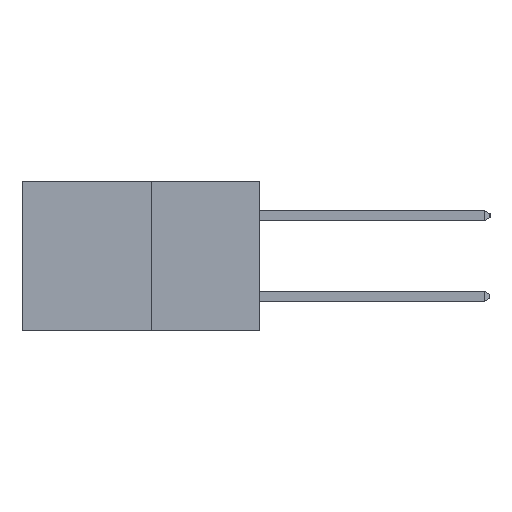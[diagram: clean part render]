
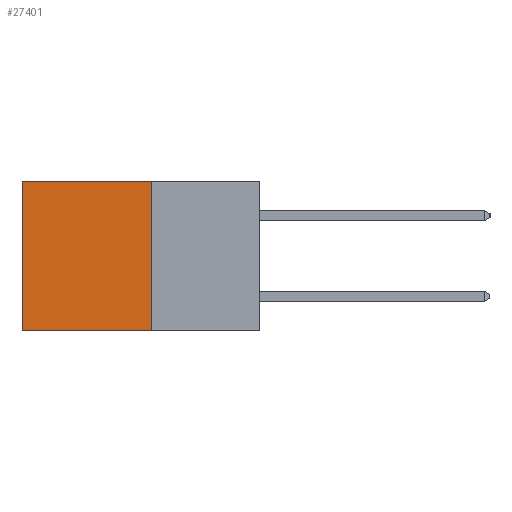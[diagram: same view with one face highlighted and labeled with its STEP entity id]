
A CAD part, left-side view. The second image highlights one B-rep face of the part: STEP entity #27401.
In plain terms, the highlighted planar face has unit normal (-1, 0, 0).
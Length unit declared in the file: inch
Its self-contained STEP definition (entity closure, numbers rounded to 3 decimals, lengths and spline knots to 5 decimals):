
#1389 = ORIENTED_EDGE ( 'NONE', *, *, #20320, .F. ) ;
#1554 = DIRECTION ( 'NONE',  ( 0., 1., 0. ) ) ;
#1926 = LINE ( 'NONE', #14057, #13884 ) ;
#4240 = VECTOR ( 'NONE', #11880, 39.37008 ) ;
#4952 = LINE ( 'NONE', #20807, #4240 ) ;
#5075 = PLANE ( 'NONE',  #5149 ) ;
#5149 = AXIS2_PLACEMENT_3D ( 'NONE', #11861, #27160, #14098 ) ;
#5764 = ORIENTED_EDGE ( 'NONE', *, *, #26866, .F. ) ;
#6046 = VERTEX_POINT ( 'NONE', #28286 ) ;
#6085 = VECTOR ( 'NONE', #18260, 39.37008 ) ;
#6684 = FACE_OUTER_BOUND ( 'NONE', #10278, .T. ) ;
#7039 = CARTESIAN_POINT ( 'NONE',  ( 0.277, 0.59, -0.37 ) ) ;
#7413 = ORIENTED_EDGE ( 'NONE', *, *, #8857, .T. ) ;
#8438 = CARTESIAN_POINT ( 'NONE',  ( 0.277, 0.27, -0.37 ) ) ;
#8534 = LINE ( 'NONE', #12747, #25444 ) ;
#8857 = EDGE_CURVE ( 'NONE', #6046, #27355, #23800, .T. ) ;
#10278 = EDGE_LOOP ( 'NONE', ( #7413, #5764, #1389, #13287 ) ) ;
#11563 = CARTESIAN_POINT ( 'NONE',  ( 0.277, 0.59, -0.37 ) ) ;
#11861 = CARTESIAN_POINT ( 'NONE',  ( 0.277, 0.27, -0.37 ) ) ;
#11880 = DIRECTION ( 'NONE',  ( 0., 1., 0. ) ) ;
#12747 = CARTESIAN_POINT ( 'NONE',  ( 0.277, 0.27, 0. ) ) ;
#13287 = ORIENTED_EDGE ( 'NONE', *, *, #16490, .T. ) ;
#13342 = VERTEX_POINT ( 'NONE', #8438 ) ;
#13884 = VECTOR ( 'NONE', #27122, 39.37008 ) ;
#14057 = CARTESIAN_POINT ( 'NONE',  ( 0.277, 0.27, -0.37 ) ) ;
#14098 = DIRECTION ( 'NONE',  ( 0., 0., -1. ) ) ;
#16490 = EDGE_CURVE ( 'NONE', #28045, #6046, #8534, .T. ) ;
#18260 = DIRECTION ( 'NONE',  ( 0., 0., -1. ) ) ;
#20320 = EDGE_CURVE ( 'NONE', #28045, #13342, #1926, .T. ) ;
#20807 = CARTESIAN_POINT ( 'NONE',  ( 0.277, 0.27, -0.37 ) ) ;
#23800 = LINE ( 'NONE', #7039, #6085 ) ;
#25444 = VECTOR ( 'NONE', #1554, 39.37008 ) ;
#26053 = CARTESIAN_POINT ( 'NONE',  ( 0.277, 0.27, 0. ) ) ;
#26866 = EDGE_CURVE ( 'NONE', #13342, #27355, #4952, .T. ) ;
#27122 = DIRECTION ( 'NONE',  ( 0., 0., -1. ) ) ;
#27160 = DIRECTION ( 'NONE',  ( 1., 0., 0. ) ) ;
#27355 = VERTEX_POINT ( 'NONE', #11563 ) ;
#27401 = ADVANCED_FACE ( 'NONE', ( #6684 ), #5075, .F. ) ;
#28045 = VERTEX_POINT ( 'NONE', #26053 ) ;
#28286 = CARTESIAN_POINT ( 'NONE',  ( 0.277, 0.59, 0. ) ) ;
